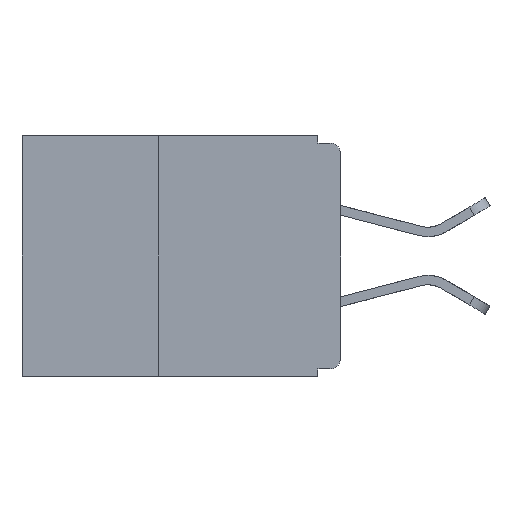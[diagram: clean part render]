
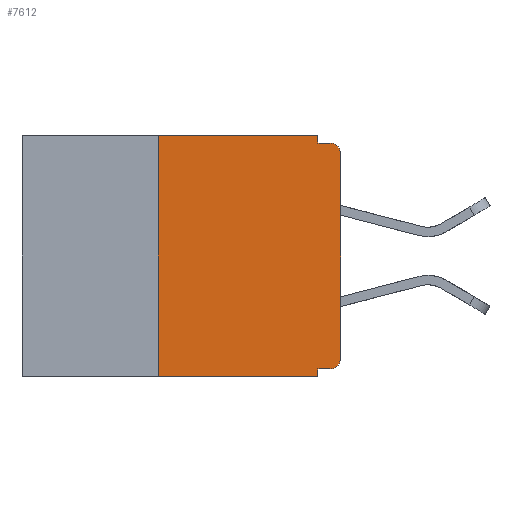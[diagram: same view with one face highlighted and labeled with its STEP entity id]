
A CAD part, left-side view. The second image highlights one B-rep face of the part: STEP entity #7612.
In plain terms, the highlighted planar face has unit normal (-1, 0, 0).
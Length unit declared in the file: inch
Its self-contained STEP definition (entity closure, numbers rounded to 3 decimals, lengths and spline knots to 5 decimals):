
#218 = VECTOR ( 'NONE', #10001, 39.37008 ) ;
#256 = EDGE_CURVE ( 'NONE', #26325, #7091, #18893, .T. ) ;
#537 = EDGE_CURVE ( 'NONE', #751, #4141, #8215, .T. ) ;
#751 = VERTEX_POINT ( 'NONE', #19761 ) ;
#878 = EDGE_CURVE ( 'NONE', #7091, #12665, #19804, .T. ) ;
#1474 = DIRECTION ( 'NONE',  ( 0., 1., 0. ) ) ;
#2720 = EDGE_CURVE ( 'NONE', #24949, #16985, #23618, .T. ) ;
#4141 = VERTEX_POINT ( 'NONE', #16858 ) ;
#4321 = CARTESIAN_POINT ( 'NONE',  ( 0., 0.25, -0.33 ) ) ;
#4422 = ORIENTED_EDGE ( 'NONE', *, *, #2720, .T. ) ;
#4493 = CARTESIAN_POINT ( 'NONE',  ( 0., 0., -0.01 ) ) ;
#4669 = CARTESIAN_POINT ( 'NONE',  ( 0., 0.031, 0. ) ) ;
#4881 = AXIS2_PLACEMENT_3D ( 'NONE', #11099, #11144, #10958 ) ;
#5757 = AXIS2_PLACEMENT_3D ( 'NONE', #19993, #22096, #19674 ) ;
#5791 = CARTESIAN_POINT ( 'NONE',  ( 0., 0.031, -0.01 ) ) ;
#6007 = ORIENTED_EDGE ( 'NONE', *, *, #256, .F. ) ;
#6374 = DIRECTION ( 'NONE',  ( 0., 0., -1. ) ) ;
#6638 = EDGE_CURVE ( 'NONE', #16985, #751, #13768, .T. ) ;
#7091 = VERTEX_POINT ( 'NONE', #17395 ) ;
#7612 = ADVANCED_FACE ( 'NONE', ( #17273 ), #11041, .F. ) ;
#7625 = CARTESIAN_POINT ( 'NONE',  ( 0., 0., -0.32 ) ) ;
#8016 = CARTESIAN_POINT ( 'NONE',  ( 0., 0., -0.305 ) ) ;
#8215 = CIRCLE ( 'NONE', #5757, 0.015 ) ;
#8295 = ORIENTED_EDGE ( 'NONE', *, *, #6638, .T. ) ;
#8629 = ORIENTED_EDGE ( 'NONE', *, *, #13828, .F. ) ;
#8826 = VECTOR ( 'NONE', #8848, 39.37008 ) ;
#8848 = DIRECTION ( 'NONE',  ( 0., -1., 0. ) ) ;
#8933 = VECTOR ( 'NONE', #23341, 39.37008 ) ;
#10001 = DIRECTION ( 'NONE',  ( 0., 0., -1. ) ) ;
#10069 = VECTOR ( 'NONE', #1474, 39.37008 ) ;
#10197 = ORIENTED_EDGE ( 'NONE', *, *, #14706, .F. ) ;
#10566 = LINE ( 'NONE', #24357, #218 ) ;
#10702 = LINE ( 'NONE', #7625, #10069 ) ;
#10766 = EDGE_CURVE ( 'NONE', #12665, #21371, #19169, .T. ) ;
#10958 = DIRECTION ( 'NONE',  ( 0., 0., -1. ) ) ;
#11041 = PLANE ( 'NONE',  #4881 ) ;
#11099 = CARTESIAN_POINT ( 'NONE',  ( 0., 0.437, 0. ) ) ;
#11144 = DIRECTION ( 'NONE',  ( 1., 0., 0. ) ) ;
#12665 = VERTEX_POINT ( 'NONE', #4669 ) ;
#13359 = VECTOR ( 'NONE', #14850, 39.37008 ) ;
#13415 = VERTEX_POINT ( 'NONE', #25085 ) ;
#13653 = VECTOR ( 'NONE', #6374, 39.37008 ) ;
#13768 = LINE ( 'NONE', #23443, #8933 ) ;
#13828 = EDGE_CURVE ( 'NONE', #14597, #13415, #10566, .T. ) ;
#14089 = ORIENTED_EDGE ( 'NONE', *, *, #15045, .F. ) ;
#14286 = EDGE_LOOP ( 'NONE', ( #8295, #25900, #10197, #15699, #21831, #6007, #17645, #8629, #14089, #4422 ) ) ;
#14597 = VERTEX_POINT ( 'NONE', #26621 ) ;
#14706 = EDGE_CURVE ( 'NONE', #21371, #4141, #19163, .T. ) ;
#14759 = CARTESIAN_POINT ( 'NONE',  ( 0., 0.25, -0.33 ) ) ;
#14850 = DIRECTION ( 'NONE',  ( 0., 0., 1. ) ) ;
#14952 = CARTESIAN_POINT ( 'NONE',  ( 0., 0.437, -0.33 ) ) ;
#15045 = EDGE_CURVE ( 'NONE', #24949, #14597, #10702, .T. ) ;
#15699 = ORIENTED_EDGE ( 'NONE', *, *, #10766, .F. ) ;
#16037 = CARTESIAN_POINT ( 'NONE',  ( 0., 0.015, -0.32 ) ) ;
#16304 = VECTOR ( 'NONE', #25118, 39.37008 ) ;
#16559 = DIRECTION ( 'NONE',  ( 0., 0., -1. ) ) ;
#16587 = DIRECTION ( 'NONE',  ( -1., 0., 0. ) ) ;
#16777 = CARTESIAN_POINT ( 'NONE',  ( 0., 0.015, -0.305 ) ) ;
#16845 = DIRECTION ( 'NONE',  ( 0., -1., 0. ) ) ;
#16858 = CARTESIAN_POINT ( 'NONE',  ( 0., 0.015, -0.01 ) ) ;
#16985 = VERTEX_POINT ( 'NONE', #8016 ) ;
#17273 = FACE_OUTER_BOUND ( 'NONE', #14286, .T. ) ;
#17395 = CARTESIAN_POINT ( 'NONE',  ( 0., 0.25, 0. ) ) ;
#17645 = ORIENTED_EDGE ( 'NONE', *, *, #23435, .T. ) ;
#18893 = LINE ( 'NONE', #14759, #13359 ) ;
#19163 = LINE ( 'NONE', #4493, #23281 ) ;
#19169 = LINE ( 'NONE', #24858, #13653 ) ;
#19674 = DIRECTION ( 'NONE',  ( 0., 0., -1. ) ) ;
#19761 = CARTESIAN_POINT ( 'NONE',  ( 0., 0., -0.025 ) ) ;
#19804 = LINE ( 'NONE', #21024, #8826 ) ;
#19993 = CARTESIAN_POINT ( 'NONE',  ( 0., 0.015, -0.025 ) ) ;
#20551 = AXIS2_PLACEMENT_3D ( 'NONE', #16777, #16587, #16559 ) ;
#21024 = CARTESIAN_POINT ( 'NONE',  ( 0., 0.437, 0. ) ) ;
#21371 = VERTEX_POINT ( 'NONE', #5791 ) ;
#21777 = LINE ( 'NONE', #14952, #16304 ) ;
#21831 = ORIENTED_EDGE ( 'NONE', *, *, #878, .F. ) ;
#22096 = DIRECTION ( 'NONE',  ( -1., 0., 0. ) ) ;
#23281 = VECTOR ( 'NONE', #16845, 39.37008 ) ;
#23341 = DIRECTION ( 'NONE',  ( 0., 0., 1. ) ) ;
#23435 = EDGE_CURVE ( 'NONE', #26325, #13415, #21777, .T. ) ;
#23443 = CARTESIAN_POINT ( 'NONE',  ( 0., 0., 0. ) ) ;
#23618 = CIRCLE ( 'NONE', #20551, 0.015 ) ;
#24357 = CARTESIAN_POINT ( 'NONE',  ( 0., 0.031, -0.33 ) ) ;
#24858 = CARTESIAN_POINT ( 'NONE',  ( 0., 0.031, 0. ) ) ;
#24949 = VERTEX_POINT ( 'NONE', #16037 ) ;
#25085 = CARTESIAN_POINT ( 'NONE',  ( 0., 0.031, -0.33 ) ) ;
#25118 = DIRECTION ( 'NONE',  ( 0., -1., 0. ) ) ;
#25900 = ORIENTED_EDGE ( 'NONE', *, *, #537, .T. ) ;
#26325 = VERTEX_POINT ( 'NONE', #4321 ) ;
#26621 = CARTESIAN_POINT ( 'NONE',  ( 0., 0.031, -0.32 ) ) ;
